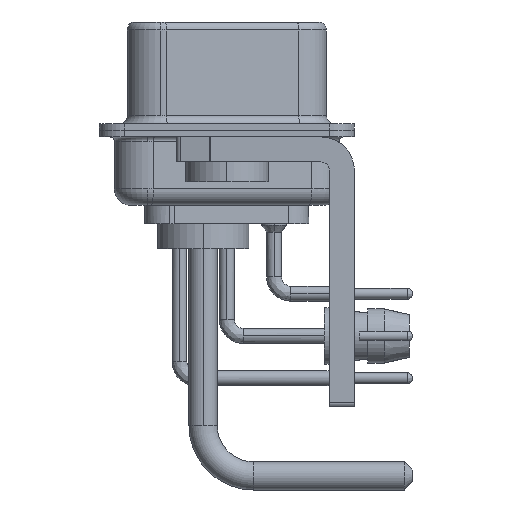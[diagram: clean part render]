
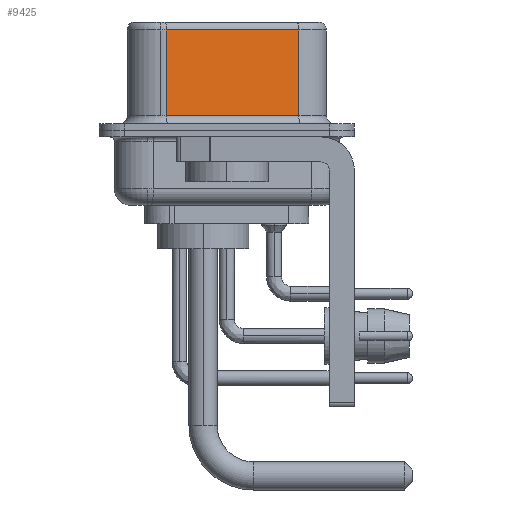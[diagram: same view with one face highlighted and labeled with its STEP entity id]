
A CAD part, left-side view. The second image highlights one B-rep face of the part: STEP entity #9425.
In plain terms, the highlighted planar face has unit normal (-0.985, -0.174, 0).
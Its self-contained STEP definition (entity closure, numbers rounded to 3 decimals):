
#467 = DIRECTION ( 'NONE',  ( -0.174, 0.985, 0. ) ) ;
#4285 = EDGE_CURVE ( 'NONE', #9566, #6598, #14903, .T. ) ;
#5439 = PLANE ( 'NONE',  #20977 ) ;
#6598 = VERTEX_POINT ( 'NONE', #18619 ) ;
#7032 = LINE ( 'NONE', #24309, #28204 ) ;
#8408 = DIRECTION ( 'NONE',  ( -0.174, 0.985, 0. ) ) ;
#9425 = ADVANCED_FACE ( 'NONE', ( #22522 ), #5439, .F. ) ;
#9539 = CARTESIAN_POINT ( 'NONE',  ( 3.73, 3.628, 0.9 ) ) ;
#9566 = VERTEX_POINT ( 'NONE', #23262 ) ;
#10156 = ORIENTED_EDGE ( 'NONE', *, *, #19866, .T. ) ;
#10997 = CARTESIAN_POINT ( 'NONE',  ( 5.132, -4.322, 0.9 ) ) ;
#11939 = CARTESIAN_POINT ( 'NONE',  ( 5.132, -4.322, 6.52 ) ) ;
#12475 = DIRECTION ( 'NONE',  ( 0., 0., -1. ) ) ;
#14903 = LINE ( 'NONE', #11939, #32137 ) ;
#16164 = VERTEX_POINT ( 'NONE', #9539 ) ;
#16949 = VERTEX_POINT ( 'NONE', #24087 ) ;
#17159 = DIRECTION ( 'NONE',  ( 0.985, 0.174, 0. ) ) ;
#17391 = CARTESIAN_POINT ( 'NONE',  ( 5.132, -4.322, 6.02 ) ) ;
#18619 = CARTESIAN_POINT ( 'NONE',  ( 5.132, -4.322, 0.9 ) ) ;
#19866 = EDGE_CURVE ( 'NONE', #9566, #16949, #31335, .T. ) ;
#20186 = ORIENTED_EDGE ( 'NONE', *, *, #35454, .T. ) ;
#20977 = AXIS2_PLACEMENT_3D ( 'NONE', #22902, #17159, #8408 ) ;
#21150 = ORIENTED_EDGE ( 'NONE', *, *, #4285, .F. ) ;
#21663 = ORIENTED_EDGE ( 'NONE', *, *, #26104, .T. ) ;
#22522 = FACE_OUTER_BOUND ( 'NONE', #32823, .T. ) ;
#22902 = CARTESIAN_POINT ( 'NONE',  ( 5.132, -4.322, 6.52 ) ) ;
#23262 = CARTESIAN_POINT ( 'NONE',  ( 5.132, -4.322, 6.02 ) ) ;
#23942 = DIRECTION ( 'NONE',  ( 0., 0., -1. ) ) ;
#24087 = CARTESIAN_POINT ( 'NONE',  ( 3.73, 3.628, 6.02 ) ) ;
#24309 = CARTESIAN_POINT ( 'NONE',  ( 3.73, 3.628, 6.52 ) ) ;
#26104 = EDGE_CURVE ( 'NONE', #16164, #6598, #36485, .T. ) ;
#28204 = VECTOR ( 'NONE', #23942, 1000. ) ;
#31126 = VECTOR ( 'NONE', #33685, 1000. ) ;
#31335 = LINE ( 'NONE', #17391, #35604 ) ;
#32137 = VECTOR ( 'NONE', #12475, 1000. ) ;
#32823 = EDGE_LOOP ( 'NONE', ( #21150, #10156, #20186, #21663 ) ) ;
#33685 = DIRECTION ( 'NONE',  ( 0.174, -0.985, 0. ) ) ;
#35454 = EDGE_CURVE ( 'NONE', #16949, #16164, #7032, .T. ) ;
#35604 = VECTOR ( 'NONE', #467, 1000. ) ;
#36485 = LINE ( 'NONE', #10997, #31126 ) ;
